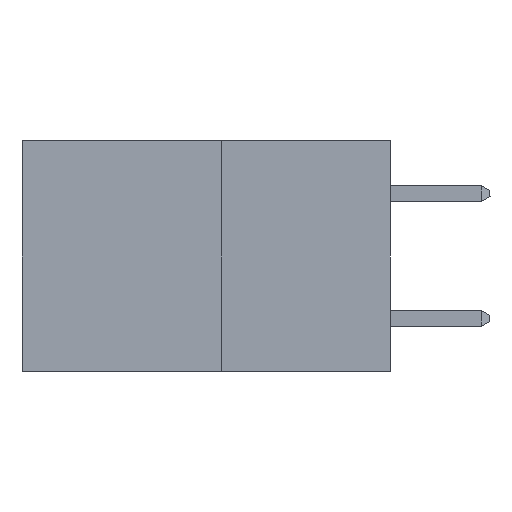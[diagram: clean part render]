
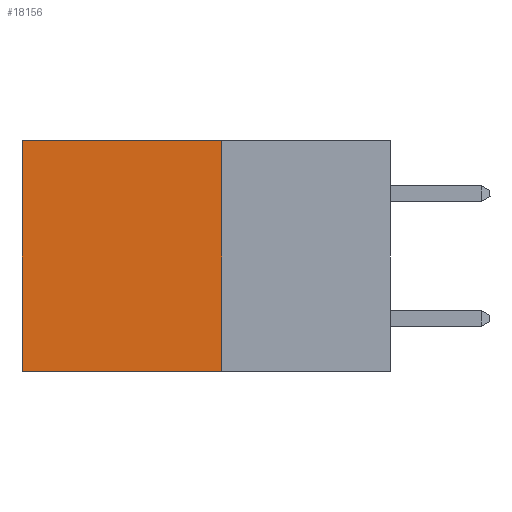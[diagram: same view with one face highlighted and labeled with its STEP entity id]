
A CAD part, left-side view. The second image highlights one B-rep face of the part: STEP entity #18156.
In plain terms, the highlighted planar face has unit normal (-1, 0, 0).
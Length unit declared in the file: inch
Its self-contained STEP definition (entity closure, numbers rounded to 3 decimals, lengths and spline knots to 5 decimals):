
#839 = DIRECTION ( 'NONE',  ( 0., 1., 0. ) ) ;
#1466 = CARTESIAN_POINT ( 'NONE',  ( 0.277, 0.59, -0.37 ) ) ;
#2411 = DIRECTION ( 'NONE',  ( 1., 0., 0. ) ) ;
#2537 = LINE ( 'NONE', #6965, #24476 ) ;
#3254 = CARTESIAN_POINT ( 'NONE',  ( 0.277, 0.59, -0.37 ) ) ;
#3396 = VECTOR ( 'NONE', #18474, 39.37008 ) ;
#4121 = AXIS2_PLACEMENT_3D ( 'NONE', #15678, #2411, #20940 ) ;
#4918 = VERTEX_POINT ( 'NONE', #14355 ) ;
#6965 = CARTESIAN_POINT ( 'NONE',  ( 0.277, 0.27, -0.37 ) ) ;
#7276 = VERTEX_POINT ( 'NONE', #29064 ) ;
#7835 = ORIENTED_EDGE ( 'NONE', *, *, #31815, .T. ) ;
#9104 = VECTOR ( 'NONE', #839, 39.37008 ) ;
#9660 = DIRECTION ( 'NONE',  ( 0., 1., 0. ) ) ;
#11007 = FACE_OUTER_BOUND ( 'NONE', #24704, .T. ) ;
#12615 = VECTOR ( 'NONE', #32273, 39.37008 ) ;
#13429 = ORIENTED_EDGE ( 'NONE', *, *, #18924, .T. ) ;
#13434 = LINE ( 'NONE', #3254, #12615 ) ;
#14355 = CARTESIAN_POINT ( 'NONE',  ( 0.277, 0.27, -0.37 ) ) ;
#14528 = ORIENTED_EDGE ( 'NONE', *, *, #30755, .F. ) ;
#15071 = CARTESIAN_POINT ( 'NONE',  ( 0.277, 0.27, 0. ) ) ;
#15678 = CARTESIAN_POINT ( 'NONE',  ( 0.277, 0.27, -0.37 ) ) ;
#16647 = VERTEX_POINT ( 'NONE', #15071 ) ;
#18156 = ADVANCED_FACE ( 'NONE', ( #11007 ), #31450, .F. ) ;
#18474 = DIRECTION ( 'NONE',  ( 0., 0., -1. ) ) ;
#18924 = EDGE_CURVE ( 'NONE', #7276, #22189, #13434, .T. ) ;
#20872 = CARTESIAN_POINT ( 'NONE',  ( 0.277, 0.27, -0.37 ) ) ;
#20940 = DIRECTION ( 'NONE',  ( 0., 0., -1. ) ) ;
#21932 = CARTESIAN_POINT ( 'NONE',  ( 0.277, 0.27, 0. ) ) ;
#22189 = VERTEX_POINT ( 'NONE', #1466 ) ;
#24476 = VECTOR ( 'NONE', #9660, 39.37008 ) ;
#24704 = EDGE_LOOP ( 'NONE', ( #13429, #14528, #30020, #7835 ) ) ;
#29064 = CARTESIAN_POINT ( 'NONE',  ( 0.277, 0.59, 0. ) ) ;
#30020 = ORIENTED_EDGE ( 'NONE', *, *, #30238, .F. ) ;
#30153 = LINE ( 'NONE', #21932, #9104 ) ;
#30238 = EDGE_CURVE ( 'NONE', #16647, #4918, #31533, .T. ) ;
#30755 = EDGE_CURVE ( 'NONE', #4918, #22189, #2537, .T. ) ;
#31450 = PLANE ( 'NONE',  #4121 ) ;
#31533 = LINE ( 'NONE', #20872, #3396 ) ;
#31815 = EDGE_CURVE ( 'NONE', #16647, #7276, #30153, .T. ) ;
#32273 = DIRECTION ( 'NONE',  ( 0., 0., -1. ) ) ;
